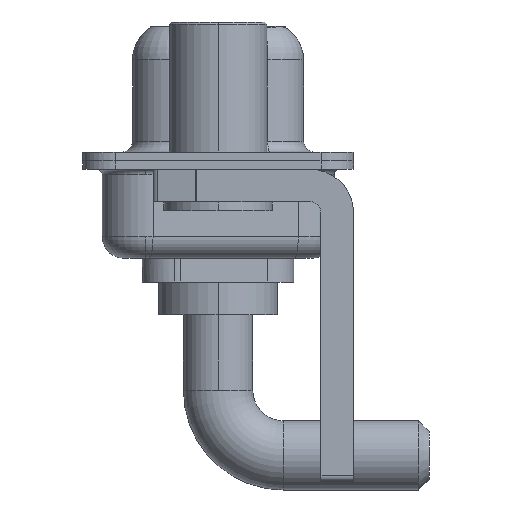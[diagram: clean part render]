
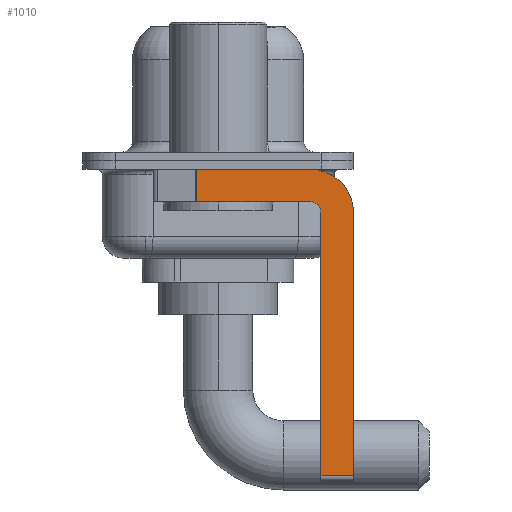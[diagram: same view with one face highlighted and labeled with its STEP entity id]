
A CAD part, left-side view. The second image highlights one B-rep face of the part: STEP entity #1010.
In plain terms, the highlighted planar face has unit normal (-1, 0, 0).
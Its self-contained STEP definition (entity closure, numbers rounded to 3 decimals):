
#39 = CARTESIAN_POINT ( 'NONE',  ( -2.9, -4.25, -14.55 ) ) ;
#109 = DIRECTION ( 'NONE',  ( 0., -1., 0. ) ) ;
#246 = CARTESIAN_POINT ( 'NONE',  ( -2.9, -4.25, -0.4 ) ) ;
#754 = VERTEX_POINT ( 'NONE', #9913 ) ;
#990 = DIRECTION ( 'NONE',  ( 0., 0., -1. ) ) ;
#1010 = ADVANCED_FACE ( 'NONE', ( #13520 ), #8853, .F. ) ;
#1195 = LINE ( 'NONE', #9023, #9605 ) ;
#1334 = CARTESIAN_POINT ( 'NONE',  ( -2.9, 0.978, -1.9 ) ) ;
#1567 = EDGE_CURVE ( 'NONE', #9570, #754, #5053, .T. ) ;
#1583 = CARTESIAN_POINT ( 'NONE',  ( -2.9, 0.978, -1.9 ) ) ;
#1589 = VECTOR ( 'NONE', #109, 1000. ) ;
#1671 = VECTOR ( 'NONE', #990, 1000. ) ;
#2281 = LINE ( 'NONE', #13875, #2515 ) ;
#2289 = ORIENTED_EDGE ( 'NONE', *, *, #10419, .F. ) ;
#2515 = VECTOR ( 'NONE', #6816, 1000. ) ;
#2657 = ORIENTED_EDGE ( 'NONE', *, *, #8418, .T. ) ;
#2666 = EDGE_LOOP ( 'NONE', ( #4348, #2657, #13629, #4454, #2289, #9916, #6533, #14024 ) ) ;
#3025 = VERTEX_POINT ( 'NONE', #6958 ) ;
#3220 = CARTESIAN_POINT ( 'NONE',  ( -2.9, -4.25, -2.4 ) ) ;
#3309 = DIRECTION ( 'NONE',  ( 0., 0., 1. ) ) ;
#3448 = DIRECTION ( 'NONE',  ( 0., 1., 0. ) ) ;
#3505 = EDGE_CURVE ( 'NONE', #11652, #13498, #11394, .T. ) ;
#4099 = AXIS2_PLACEMENT_3D ( 'NONE', #12373, #4640, #10119 ) ;
#4348 = ORIENTED_EDGE ( 'NONE', *, *, #7985, .F. ) ;
#4454 = ORIENTED_EDGE ( 'NONE', *, *, #8800, .F. ) ;
#4640 = DIRECTION ( 'NONE',  ( 1., 0., 0. ) ) ;
#4838 = DIRECTION ( 'NONE',  ( 0., 0., -1. ) ) ;
#5053 = CIRCLE ( 'NONE', #4099, 2. ) ;
#5776 = EDGE_CURVE ( 'NONE', #3025, #13548, #7063, .T. ) ;
#6258 = AXIS2_PLACEMENT_3D ( 'NONE', #3220, #6674, #14713 ) ;
#6321 = EDGE_CURVE ( 'NONE', #754, #13498, #11590, .T. ) ;
#6333 = CARTESIAN_POINT ( 'NONE',  ( -2.9, -4.75, -2.4 ) ) ;
#6463 = VECTOR ( 'NONE', #3448, 1000. ) ;
#6533 = ORIENTED_EDGE ( 'NONE', *, *, #6321, .F. ) ;
#6674 = DIRECTION ( 'NONE',  ( 1., 0., 0. ) ) ;
#6816 = DIRECTION ( 'NONE',  ( 0., -1., 0. ) ) ;
#6893 = VECTOR ( 'NONE', #4838, 1000. ) ;
#6958 = CARTESIAN_POINT ( 'NONE',  ( -2.9, -4.25, -1.9 ) ) ;
#7063 = LINE ( 'NONE', #14787, #6463 ) ;
#7304 = VERTEX_POINT ( 'NONE', #6333 ) ;
#7671 = CARTESIAN_POINT ( 'NONE',  ( -2.9, -4.25, -2.4 ) ) ;
#7985 = EDGE_CURVE ( 'NONE', #13224, #9570, #2281, .T. ) ;
#8418 = EDGE_CURVE ( 'NONE', #13224, #13548, #12423, .T. ) ;
#8510 = CARTESIAN_POINT ( 'NONE',  ( -2.9, -6.25, -14.55 ) ) ;
#8787 = DIRECTION ( 'NONE',  ( -1., 0., 0. ) ) ;
#8800 = EDGE_CURVE ( 'NONE', #7304, #3025, #14873, .T. ) ;
#8853 = PLANE ( 'NONE',  #6258 ) ;
#9023 = CARTESIAN_POINT ( 'NONE',  ( -2.9, -4.75, -14.8 ) ) ;
#9570 = VERTEX_POINT ( 'NONE', #246 ) ;
#9605 = VECTOR ( 'NONE', #3309, 1000. ) ;
#9913 = CARTESIAN_POINT ( 'NONE',  ( -2.9, -6.25, -2.4 ) ) ;
#9916 = ORIENTED_EDGE ( 'NONE', *, *, #3505, .T. ) ;
#10119 = DIRECTION ( 'NONE',  ( 0., 0., -1. ) ) ;
#10419 = EDGE_CURVE ( 'NONE', #11652, #7304, #1195, .T. ) ;
#10616 = CARTESIAN_POINT ( 'NONE',  ( -2.9, -6.25, -2.4 ) ) ;
#11394 = LINE ( 'NONE', #39, #1589 ) ;
#11590 = LINE ( 'NONE', #10616, #6893 ) ;
#11652 = VERTEX_POINT ( 'NONE', #14306 ) ;
#12373 = CARTESIAN_POINT ( 'NONE',  ( -2.9, -4.25, -2.4 ) ) ;
#12423 = LINE ( 'NONE', #1334, #1671 ) ;
#13224 = VERTEX_POINT ( 'NONE', #13557 ) ;
#13498 = VERTEX_POINT ( 'NONE', #8510 ) ;
#13520 = FACE_OUTER_BOUND ( 'NONE', #2666, .T. ) ;
#13528 = DIRECTION ( 'NONE',  ( 0., 0., 1. ) ) ;
#13548 = VERTEX_POINT ( 'NONE', #1583 ) ;
#13557 = CARTESIAN_POINT ( 'NONE',  ( -2.9, 0.978, -0.4 ) ) ;
#13629 = ORIENTED_EDGE ( 'NONE', *, *, #5776, .F. ) ;
#13875 = CARTESIAN_POINT ( 'NONE',  ( -2.9, 3., -0.4 ) ) ;
#14024 = ORIENTED_EDGE ( 'NONE', *, *, #1567, .F. ) ;
#14168 = AXIS2_PLACEMENT_3D ( 'NONE', #7671, #8787, #13528 ) ;
#14306 = CARTESIAN_POINT ( 'NONE',  ( -2.9, -4.75, -14.55 ) ) ;
#14713 = DIRECTION ( 'NONE',  ( 0., 0., -1. ) ) ;
#14787 = CARTESIAN_POINT ( 'NONE',  ( -2.9, -4.25, -1.9 ) ) ;
#14873 = CIRCLE ( 'NONE', #14168, 0.5 ) ;
